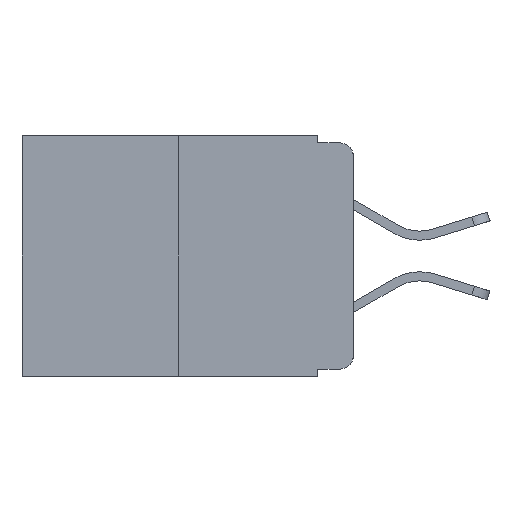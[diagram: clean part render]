
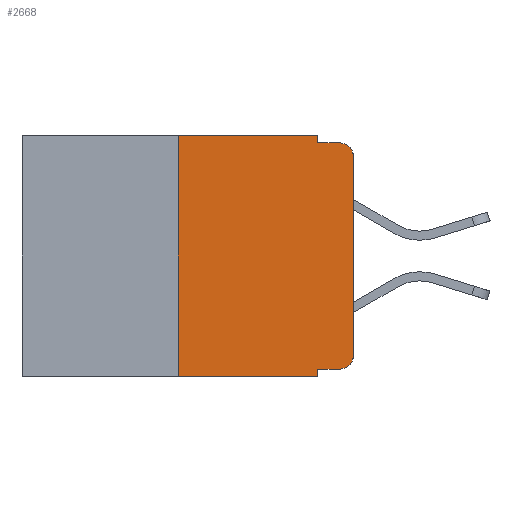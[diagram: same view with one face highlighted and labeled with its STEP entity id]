
A CAD part, left-side view. The second image highlights one B-rep face of the part: STEP entity #2668.
In plain terms, the highlighted planar face has unit normal (-1, 0, 0).
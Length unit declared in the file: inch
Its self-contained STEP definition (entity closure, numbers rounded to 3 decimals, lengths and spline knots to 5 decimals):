
#21 = CARTESIAN_POINT ( 'NONE',  ( 0., 0.02, -0.01 ) ) ;
#433 = VERTEX_POINT ( 'NONE', #9683 ) ;
#647 = LINE ( 'NONE', #17849, #14142 ) ;
#692 = ORIENTED_EDGE ( 'NONE', *, *, #1955, .F. ) ;
#1020 = EDGE_CURVE ( 'NONE', #433, #8700, #1576, .T. ) ;
#1066 = AXIS2_PLACEMENT_3D ( 'NONE', #4791, #4779, #14339 ) ;
#1077 = VERTEX_POINT ( 'NONE', #11467 ) ;
#1218 = DIRECTION ( 'NONE',  ( 0., 0., 1. ) ) ;
#1251 = AXIS2_PLACEMENT_3D ( 'NONE', #1532, #14126, #13424 ) ;
#1532 = CARTESIAN_POINT ( 'NONE',  ( 0., 0.473, 0. ) ) ;
#1576 = LINE ( 'NONE', #9970, #15045 ) ;
#1955 = EDGE_CURVE ( 'NONE', #433, #8247, #15851, .T. ) ;
#2077 = CARTESIAN_POINT ( 'NONE',  ( 0., 0.051, 0. ) ) ;
#2376 = VERTEX_POINT ( 'NONE', #21 ) ;
#2616 = CARTESIAN_POINT ( 'NONE',  ( 0., 0.473, 0. ) ) ;
#2668 = ADVANCED_FACE ( 'NONE', ( #8814 ), #6195, .F. ) ;
#2914 = DIRECTION ( 'NONE',  ( -1., 0., 0. ) ) ;
#3117 = CARTESIAN_POINT ( 'NONE',  ( 0., 0.051, -0.01 ) ) ;
#3542 = ORIENTED_EDGE ( 'NONE', *, *, #9457, .F. ) ;
#3834 = CIRCLE ( 'NONE', #1066, 0.02 ) ;
#3876 = CARTESIAN_POINT ( 'NONE',  ( 0., 0.25, 0. ) ) ;
#3979 = EDGE_LOOP ( 'NONE', ( #7110, #7539, #12023, #16085, #10063, #3542, #10934, #692, #4427, #5337 ) ) ;
#4144 = DIRECTION ( 'NONE',  ( 0., 0., 1. ) ) ;
#4210 = DIRECTION ( 'NONE',  ( 0., 0., -1. ) ) ;
#4427 = ORIENTED_EDGE ( 'NONE', *, *, #1020, .T. ) ;
#4441 = DIRECTION ( 'NONE',  ( 0., -1., 0. ) ) ;
#4779 = DIRECTION ( 'NONE',  ( -1., 0., 0. ) ) ;
#4791 = CARTESIAN_POINT ( 'NONE',  ( 0., 0.02, -0.03 ) ) ;
#4854 = VERTEX_POINT ( 'NONE', #3876 ) ;
#4875 = VERTEX_POINT ( 'NONE', #2077 ) ;
#4935 = LINE ( 'NONE', #10961, #8241 ) ;
#5337 = ORIENTED_EDGE ( 'NONE', *, *, #12582, .T. ) ;
#5894 = VERTEX_POINT ( 'NONE', #15074 ) ;
#6195 = PLANE ( 'NONE',  #1251 ) ;
#6368 = EDGE_CURVE ( 'NONE', #15601, #2376, #11460, .T. ) ;
#6554 = DIRECTION ( 'NONE',  ( 0., 0., -1. ) ) ;
#6555 = VECTOR ( 'NONE', #14621, 39.37008 ) ;
#6610 = AXIS2_PLACEMENT_3D ( 'NONE', #11234, #2914, #12638 ) ;
#6970 = EDGE_CURVE ( 'NONE', #1077, #2376, #3834, .T. ) ;
#7110 = ORIENTED_EDGE ( 'NONE', *, *, #12473, .T. ) ;
#7311 = VECTOR ( 'NONE', #4210, 39.37008 ) ;
#7378 = LINE ( 'NONE', #2616, #17810 ) ;
#7539 = ORIENTED_EDGE ( 'NONE', *, *, #6970, .T. ) ;
#8241 = VECTOR ( 'NONE', #1218, 39.37008 ) ;
#8247 = VERTEX_POINT ( 'NONE', #9397 ) ;
#8700 = VERTEX_POINT ( 'NONE', #15842 ) ;
#8814 = FACE_OUTER_BOUND ( 'NONE', #3979, .T. ) ;
#9397 = CARTESIAN_POINT ( 'NONE',  ( 0., 0.051, -0.343 ) ) ;
#9457 = EDGE_CURVE ( 'NONE', #5894, #4854, #4935, .T. ) ;
#9683 = CARTESIAN_POINT ( 'NONE',  ( 0., 0.051, -0.333 ) ) ;
#9970 = CARTESIAN_POINT ( 'NONE',  ( 0., 0.051, -0.333 ) ) ;
#10005 = DIRECTION ( 'NONE',  ( 0., -1., 0. ) ) ;
#10063 = ORIENTED_EDGE ( 'NONE', *, *, #16641, .F. ) ;
#10864 = DIRECTION ( 'NONE',  ( 0., -1., 0. ) ) ;
#10934 = ORIENTED_EDGE ( 'NONE', *, *, #17377, .T. ) ;
#10961 = CARTESIAN_POINT ( 'NONE',  ( 0., 0.25, 0. ) ) ;
#11234 = CARTESIAN_POINT ( 'NONE',  ( 0., 0.02, -0.313 ) ) ;
#11460 = LINE ( 'NONE', #14846, #6555 ) ;
#11467 = CARTESIAN_POINT ( 'NONE',  ( 0., 0., -0.03 ) ) ;
#11650 = CARTESIAN_POINT ( 'NONE',  ( 0., 0., -0.313 ) ) ;
#12023 = ORIENTED_EDGE ( 'NONE', *, *, #6368, .F. ) ;
#12473 = EDGE_CURVE ( 'NONE', #13255, #1077, #647, .T. ) ;
#12582 = EDGE_CURVE ( 'NONE', #8700, #13255, #16889, .T. ) ;
#12638 = DIRECTION ( 'NONE',  ( 0., 0., -1. ) ) ;
#13255 = VERTEX_POINT ( 'NONE', #11650 ) ;
#13424 = DIRECTION ( 'NONE',  ( 0., 0., -1. ) ) ;
#13991 = LINE ( 'NONE', #14144, #16740 ) ;
#14126 = DIRECTION ( 'NONE',  ( 1., 0., 0. ) ) ;
#14142 = VECTOR ( 'NONE', #4144, 39.37008 ) ;
#14144 = CARTESIAN_POINT ( 'NONE',  ( 0., 0.473, -0.343 ) ) ;
#14339 = DIRECTION ( 'NONE',  ( 0., 0., -1. ) ) ;
#14621 = DIRECTION ( 'NONE',  ( 0., -1., 0. ) ) ;
#14846 = CARTESIAN_POINT ( 'NONE',  ( 0., 0.051, -0.01 ) ) ;
#15045 = VECTOR ( 'NONE', #10005, 39.37008 ) ;
#15074 = CARTESIAN_POINT ( 'NONE',  ( 0., 0.25, -0.343 ) ) ;
#15601 = VERTEX_POINT ( 'NONE', #3117 ) ;
#15842 = CARTESIAN_POINT ( 'NONE',  ( 0., 0.02, -0.333 ) ) ;
#15851 = LINE ( 'NONE', #16844, #7311 ) ;
#15882 = EDGE_CURVE ( 'NONE', #4875, #15601, #17007, .T. ) ;
#16085 = ORIENTED_EDGE ( 'NONE', *, *, #15882, .F. ) ;
#16122 = CARTESIAN_POINT ( 'NONE',  ( 0., 0.051, 0. ) ) ;
#16641 = EDGE_CURVE ( 'NONE', #4854, #4875, #7378, .T. ) ;
#16740 = VECTOR ( 'NONE', #4441, 39.37008 ) ;
#16844 = CARTESIAN_POINT ( 'NONE',  ( 0., 0.051, 0. ) ) ;
#16889 = CIRCLE ( 'NONE', #6610, 0.02 ) ;
#17007 = LINE ( 'NONE', #16122, #17840 ) ;
#17377 = EDGE_CURVE ( 'NONE', #5894, #8247, #13991, .T. ) ;
#17810 = VECTOR ( 'NONE', #10864, 39.37008 ) ;
#17840 = VECTOR ( 'NONE', #6554, 39.37008 ) ;
#17849 = CARTESIAN_POINT ( 'NONE',  ( 0., 0., 0. ) ) ;
